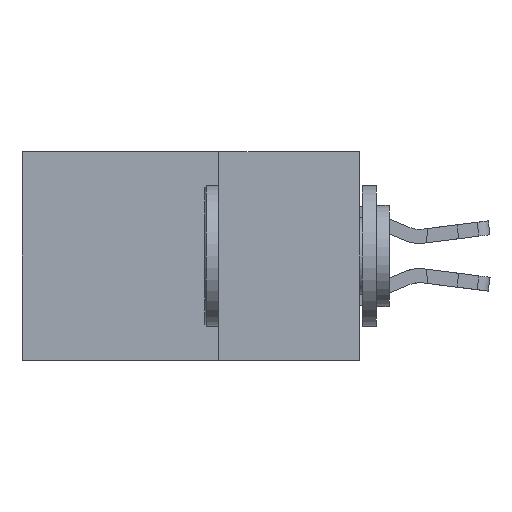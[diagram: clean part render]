
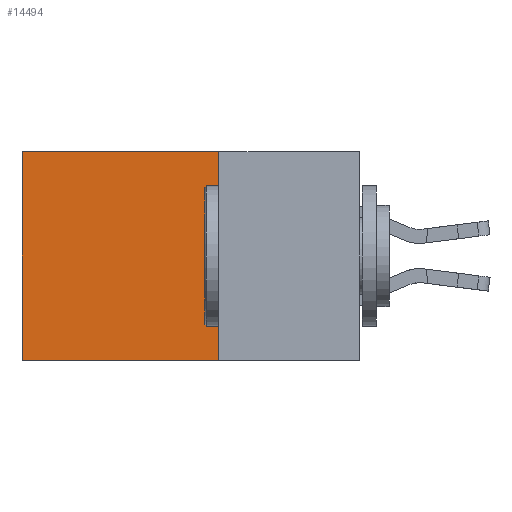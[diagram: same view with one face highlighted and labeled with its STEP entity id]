
A CAD part, left-side view. The second image highlights one B-rep face of the part: STEP entity #14494.
In plain terms, the highlighted planar face has unit normal (-1, 0, 0).
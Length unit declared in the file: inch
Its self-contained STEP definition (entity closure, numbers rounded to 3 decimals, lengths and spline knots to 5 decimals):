
#962 = CARTESIAN_POINT ( 'NONE',  ( 0.2875, 0.25, -0.37 ) ) ;
#1952 = ORIENTED_EDGE ( 'NONE', *, *, #21145, .T. ) ;
#2387 = DIRECTION ( 'NONE',  ( 0., 1., 0. ) ) ;
#4496 = ORIENTED_EDGE ( 'NONE', *, *, #7172, .F. ) ;
#4499 = DIRECTION ( 'NONE',  ( 0., 1., 0. ) ) ;
#4958 = LINE ( 'NONE', #21276, #13866 ) ;
#5407 = DIRECTION ( 'NONE',  ( 0., 0., -1. ) ) ;
#5531 = ORIENTED_EDGE ( 'NONE', *, *, #19553, .T. ) ;
#5731 = VERTEX_POINT ( 'NONE', #11735 ) ;
#5921 = CARTESIAN_POINT ( 'NONE',  ( 0.2875, 0.25, 0. ) ) ;
#6746 = CARTESIAN_POINT ( 'NONE',  ( 0.2875, 0.6, 0. ) ) ;
#6819 = EDGE_CURVE ( 'NONE', #16047, #5731, #16834, .T. ) ;
#7172 = EDGE_CURVE ( 'NONE', #20210, #16047, #4958, .T. ) ;
#7519 = VECTOR ( 'NONE', #4499, 39.37008 ) ;
#8043 = VECTOR ( 'NONE', #2387, 39.37008 ) ;
#8450 = DIRECTION ( 'NONE',  ( 0., 0., -1. ) ) ;
#8659 = EDGE_LOOP ( 'NONE', ( #1952, #12679, #4496, #5531 ) ) ;
#8904 = AXIS2_PLACEMENT_3D ( 'NONE', #21957, #9865, #22032 ) ;
#9865 = DIRECTION ( 'NONE',  ( 1., 0., 0. ) ) ;
#11095 = LINE ( 'NONE', #20683, #14597 ) ;
#11335 = CARTESIAN_POINT ( 'NONE',  ( 0.2875, 0.25, 0. ) ) ;
#11735 = CARTESIAN_POINT ( 'NONE',  ( 0.2875, 0.6, -0.37 ) ) ;
#12679 = ORIENTED_EDGE ( 'NONE', *, *, #6819, .F. ) ;
#13866 = VECTOR ( 'NONE', #5407, 39.37008 ) ;
#14494 = ADVANCED_FACE ( 'NONE', ( #16270 ), #20287, .F. ) ;
#14597 = VECTOR ( 'NONE', #8450, 39.37008 ) ;
#16047 = VERTEX_POINT ( 'NONE', #18236 ) ;
#16270 = FACE_OUTER_BOUND ( 'NONE', #8659, .T. ) ;
#16834 = LINE ( 'NONE', #962, #7519 ) ;
#17909 = LINE ( 'NONE', #5921, #8043 ) ;
#18236 = CARTESIAN_POINT ( 'NONE',  ( 0.2875, 0.25, -0.37 ) ) ;
#19553 = EDGE_CURVE ( 'NONE', #20210, #19854, #17909, .T. ) ;
#19854 = VERTEX_POINT ( 'NONE', #6746 ) ;
#20210 = VERTEX_POINT ( 'NONE', #11335 ) ;
#20287 = PLANE ( 'NONE',  #8904 ) ;
#20683 = CARTESIAN_POINT ( 'NONE',  ( 0.2875, 0.6, 0. ) ) ;
#21145 = EDGE_CURVE ( 'NONE', #19854, #5731, #11095, .T. ) ;
#21276 = CARTESIAN_POINT ( 'NONE',  ( 0.2875, 0.25, 0. ) ) ;
#21957 = CARTESIAN_POINT ( 'NONE',  ( 0.2875, 0.25, 0. ) ) ;
#22032 = DIRECTION ( 'NONE',  ( 0., 0., -1. ) ) ;
